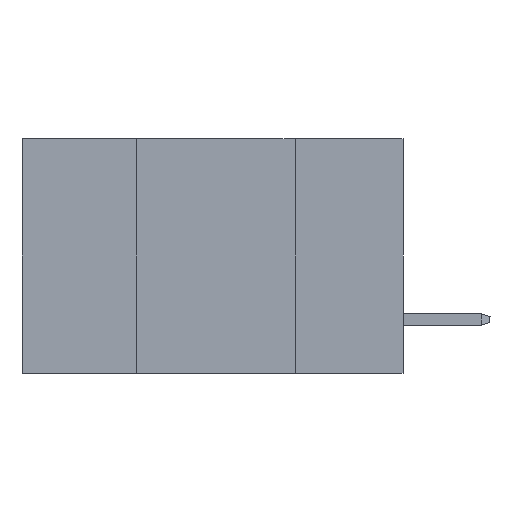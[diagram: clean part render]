
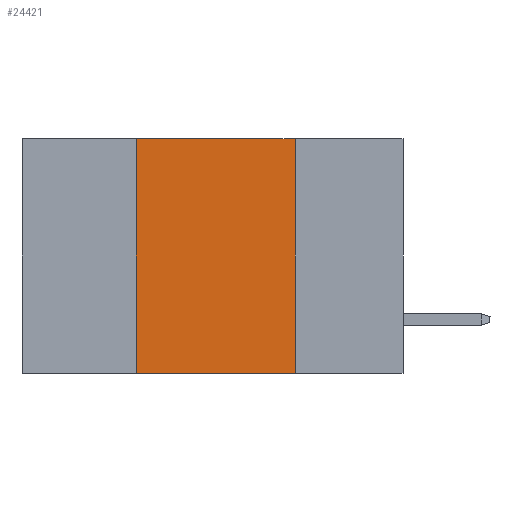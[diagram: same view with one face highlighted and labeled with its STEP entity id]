
A CAD part, left-side view. The second image highlights one B-rep face of the part: STEP entity #24421.
In plain terms, the highlighted planar face has unit normal (-1, 0, 0).
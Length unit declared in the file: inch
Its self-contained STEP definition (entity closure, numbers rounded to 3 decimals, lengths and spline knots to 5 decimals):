
#770 = DIRECTION ( 'NONE',  ( 0., -1., 0. ) ) ;
#794 = PLANE ( 'NONE',  #15075 ) ;
#1015 = DIRECTION ( 'NONE',  ( 0., -1., 0. ) ) ;
#1549 = VECTOR ( 'NONE', #25164, 39.37008 ) ;
#2259 = CARTESIAN_POINT ( 'NONE',  ( 0., 0.42, 0. ) ) ;
#2315 = CARTESIAN_POINT ( 'NONE',  ( 0., 0.42, -0.37 ) ) ;
#4715 = EDGE_CURVE ( 'NONE', #12854, #12524, #9675, .T. ) ;
#5081 = DIRECTION ( 'NONE',  ( 0., 0., 1. ) ) ;
#5082 = FACE_OUTER_BOUND ( 'NONE', #10560, .T. ) ;
#5774 = VECTOR ( 'NONE', #5081, 39.37008 ) ;
#6224 = VERTEX_POINT ( 'NONE', #10916 ) ;
#7933 = CARTESIAN_POINT ( 'NONE',  ( 0., 0.6, 0. ) ) ;
#8086 = DIRECTION ( 'NONE',  ( 0., 0., -1. ) ) ;
#8791 = EDGE_CURVE ( 'NONE', #6224, #14259, #27077, .T. ) ;
#9675 = LINE ( 'NONE', #2259, #5774 ) ;
#10522 = ORIENTED_EDGE ( 'NONE', *, *, #4715, .F. ) ;
#10560 = EDGE_LOOP ( 'NONE', ( #26539, #18407, #10522, #14163 ) ) ;
#10916 = CARTESIAN_POINT ( 'NONE',  ( 0., 0.17, 0. ) ) ;
#11893 = VECTOR ( 'NONE', #1015, 39.37008 ) ;
#12524 = VERTEX_POINT ( 'NONE', #16325 ) ;
#12854 = VERTEX_POINT ( 'NONE', #2315 ) ;
#12876 = CARTESIAN_POINT ( 'NONE',  ( 0., 0.17, 0. ) ) ;
#12961 = EDGE_CURVE ( 'NONE', #12524, #6224, #17618, .T. ) ;
#14163 = ORIENTED_EDGE ( 'NONE', *, *, #17377, .T. ) ;
#14259 = VERTEX_POINT ( 'NONE', #16645 ) ;
#15075 = AXIS2_PLACEMENT_3D ( 'NONE', #7933, #26893, #8086 ) ;
#16325 = CARTESIAN_POINT ( 'NONE',  ( 0., 0.42, 0. ) ) ;
#16645 = CARTESIAN_POINT ( 'NONE',  ( 0., 0.17, -0.37 ) ) ;
#17377 = EDGE_CURVE ( 'NONE', #12854, #14259, #17997, .T. ) ;
#17618 = LINE ( 'NONE', #29468, #11893 ) ;
#17997 = LINE ( 'NONE', #18158, #31023 ) ;
#18158 = CARTESIAN_POINT ( 'NONE',  ( 0., 0.6, -0.37 ) ) ;
#18407 = ORIENTED_EDGE ( 'NONE', *, *, #12961, .F. ) ;
#24421 = ADVANCED_FACE ( 'NONE', ( #5082 ), #794, .F. ) ;
#25164 = DIRECTION ( 'NONE',  ( 0., 0., -1. ) ) ;
#26539 = ORIENTED_EDGE ( 'NONE', *, *, #8791, .F. ) ;
#26893 = DIRECTION ( 'NONE',  ( 1., 0., 0. ) ) ;
#27077 = LINE ( 'NONE', #12876, #1549 ) ;
#29468 = CARTESIAN_POINT ( 'NONE',  ( 0., 0.6, 0. ) ) ;
#31023 = VECTOR ( 'NONE', #770, 39.37008 ) ;
